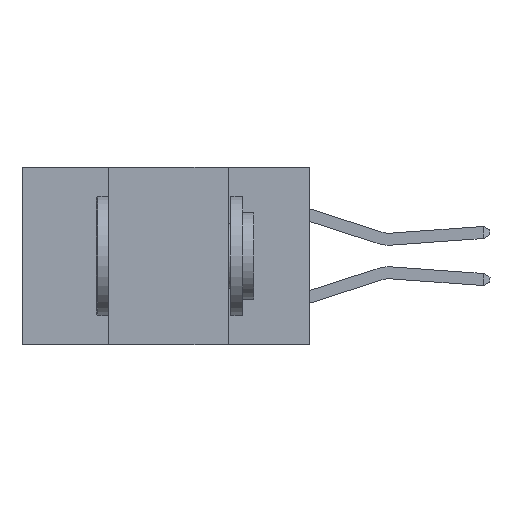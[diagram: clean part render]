
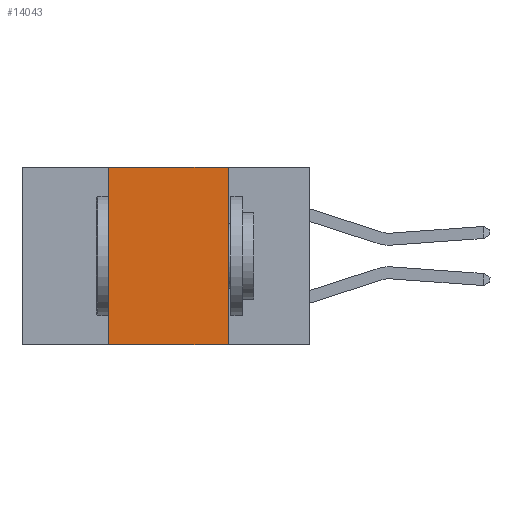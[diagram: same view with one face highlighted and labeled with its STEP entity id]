
A CAD part, left-side view. The second image highlights one B-rep face of the part: STEP entity #14043.
In plain terms, the highlighted planar face has unit normal (-1, 0, 0).
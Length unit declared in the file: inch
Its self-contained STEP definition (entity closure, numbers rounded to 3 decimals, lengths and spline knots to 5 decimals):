
#1020 = EDGE_CURVE ( 'NONE', #10737, #14430, #16788, .T. ) ;
#1458 = DIRECTION ( 'NONE',  ( 0., 0., 1. ) ) ;
#1571 = CARTESIAN_POINT ( 'NONE',  ( 0., 0.42, 0. ) ) ;
#1786 = EDGE_LOOP ( 'NONE', ( #6655, #7345, #7813, #8641 ) ) ;
#3827 = VECTOR ( 'NONE', #19086, 39.37008 ) ;
#4099 = CARTESIAN_POINT ( 'NONE',  ( 0., 0.17, 0. ) ) ;
#6655 = ORIENTED_EDGE ( 'NONE', *, *, #21208, .F. ) ;
#7287 = PLANE ( 'NONE',  #17190 ) ;
#7345 = ORIENTED_EDGE ( 'NONE', *, *, #19214, .F. ) ;
#7813 = ORIENTED_EDGE ( 'NONE', *, *, #1020, .F. ) ;
#7994 = VECTOR ( 'NONE', #30879, 39.37008 ) ;
#8641 = ORIENTED_EDGE ( 'NONE', *, *, #9078, .T. ) ;
#9078 = EDGE_CURVE ( 'NONE', #10737, #27325, #10689, .T. ) ;
#9807 = DIRECTION ( 'NONE',  ( 0., 0., -1. ) ) ;
#10689 = LINE ( 'NONE', #21916, #16516 ) ;
#10737 = VERTEX_POINT ( 'NONE', #30413 ) ;
#11208 = CARTESIAN_POINT ( 'NONE',  ( 0., 0.6, 0. ) ) ;
#11495 = FACE_OUTER_BOUND ( 'NONE', #1786, .T. ) ;
#14043 = ADVANCED_FACE ( 'NONE', ( #11495 ), #7287, .F. ) ;
#14430 = VERTEX_POINT ( 'NONE', #28491 ) ;
#16186 = LINE ( 'NONE', #11208, #7994 ) ;
#16516 = VECTOR ( 'NONE', #29255, 39.37008 ) ;
#16788 = LINE ( 'NONE', #1571, #23433 ) ;
#17190 = AXIS2_PLACEMENT_3D ( 'NONE', #17218, #24715, #9807 ) ;
#17218 = CARTESIAN_POINT ( 'NONE',  ( 0., 0.6, 0. ) ) ;
#17545 = VERTEX_POINT ( 'NONE', #20564 ) ;
#19086 = DIRECTION ( 'NONE',  ( 0., 0., -1. ) ) ;
#19214 = EDGE_CURVE ( 'NONE', #14430, #17545, #16186, .T. ) ;
#20564 = CARTESIAN_POINT ( 'NONE',  ( 0., 0.17, 0. ) ) ;
#21208 = EDGE_CURVE ( 'NONE', #17545, #27325, #23771, .T. ) ;
#21916 = CARTESIAN_POINT ( 'NONE',  ( 0., 0.6, -0.37 ) ) ;
#23433 = VECTOR ( 'NONE', #1458, 39.37008 ) ;
#23771 = LINE ( 'NONE', #4099, #3827 ) ;
#24464 = CARTESIAN_POINT ( 'NONE',  ( 0., 0.17, -0.37 ) ) ;
#24715 = DIRECTION ( 'NONE',  ( 1., 0., 0. ) ) ;
#27325 = VERTEX_POINT ( 'NONE', #24464 ) ;
#28491 = CARTESIAN_POINT ( 'NONE',  ( 0., 0.42, 0. ) ) ;
#29255 = DIRECTION ( 'NONE',  ( 0., -1., 0. ) ) ;
#30413 = CARTESIAN_POINT ( 'NONE',  ( 0., 0.42, -0.37 ) ) ;
#30879 = DIRECTION ( 'NONE',  ( 0., -1., 0. ) ) ;
